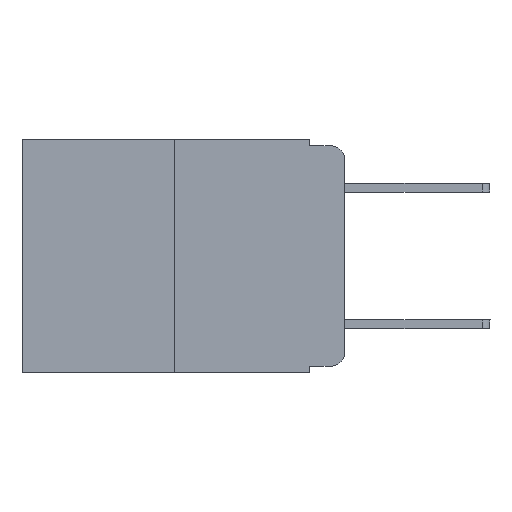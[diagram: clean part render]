
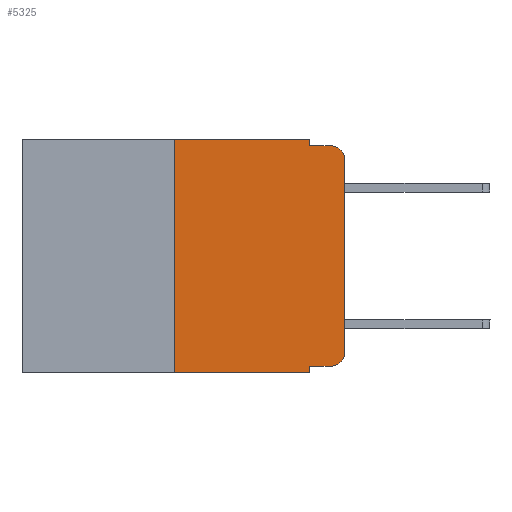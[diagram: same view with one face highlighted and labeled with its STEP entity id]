
A CAD part, left-side view. The second image highlights one B-rep face of the part: STEP entity #5325.
In plain terms, the highlighted planar face has unit normal (-1, 0, 0).
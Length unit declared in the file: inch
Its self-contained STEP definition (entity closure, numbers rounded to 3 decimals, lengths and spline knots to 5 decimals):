
#109 = DIRECTION ( 'NONE',  ( 0., 0., -1. ) ) ;
#669 = DIRECTION ( 'NONE',  ( 1., 0., 0. ) ) ;
#818 = DIRECTION ( 'NONE',  ( -1., 0., 0. ) ) ;
#1307 = AXIS2_PLACEMENT_3D ( 'NONE', #4629, #669, #14465 ) ;
#1633 = DIRECTION ( 'NONE',  ( 0., 0., 1. ) ) ;
#1715 = CARTESIAN_POINT ( 'NONE',  ( 0., 0.25, 0. ) ) ;
#1912 = EDGE_CURVE ( 'NONE', #17493, #9407, #16410, .T. ) ;
#2151 = AXIS2_PLACEMENT_3D ( 'NONE', #16665, #11224, #109 ) ;
#2293 = EDGE_CURVE ( 'NONE', #14883, #9252, #6086, .T. ) ;
#2622 = ORIENTED_EDGE ( 'NONE', *, *, #1912, .T. ) ;
#2721 = VERTEX_POINT ( 'NONE', #11916 ) ;
#2787 = DIRECTION ( 'NONE',  ( 0., -1., 0. ) ) ;
#2846 = VECTOR ( 'NONE', #4198, 39.37008 ) ;
#2857 = ORIENTED_EDGE ( 'NONE', *, *, #6611, .F. ) ;
#3054 = CARTESIAN_POINT ( 'NONE',  ( 0., 0.051, -0.343 ) ) ;
#3123 = LINE ( 'NONE', #12348, #15602 ) ;
#3141 = EDGE_CURVE ( 'NONE', #12394, #9407, #14872, .T. ) ;
#3648 = DIRECTION ( 'NONE',  ( 0., -1., 0. ) ) ;
#3745 = CARTESIAN_POINT ( 'NONE',  ( 0., 0.02, -0.333 ) ) ;
#3758 = VERTEX_POINT ( 'NONE', #16646 ) ;
#3773 = CARTESIAN_POINT ( 'NONE',  ( 0., 0.051, -0.333 ) ) ;
#4007 = DIRECTION ( 'NONE',  ( 0., -1., 0. ) ) ;
#4198 = DIRECTION ( 'NONE',  ( 0., 0., 1. ) ) ;
#4251 = CARTESIAN_POINT ( 'NONE',  ( 0., 0.051, -0.01 ) ) ;
#4394 = LINE ( 'NONE', #17704, #8910 ) ;
#4629 = CARTESIAN_POINT ( 'NONE',  ( 0., 0.473, 0. ) ) ;
#4828 = VECTOR ( 'NONE', #2787, 39.37008 ) ;
#4903 = DIRECTION ( 'NONE',  ( 0., 0., -1. ) ) ;
#4929 = CARTESIAN_POINT ( 'NONE',  ( 0., 0.02, -0.03 ) ) ;
#5201 = VERTEX_POINT ( 'NONE', #3054 ) ;
#5233 = CARTESIAN_POINT ( 'NONE',  ( 0., 0., -0.313 ) ) ;
#5248 = DIRECTION ( 'NONE',  ( 0., 0., -1. ) ) ;
#5325 = ADVANCED_FACE ( 'NONE', ( #15027 ), #16827, .F. ) ;
#6073 = VECTOR ( 'NONE', #4903, 39.37008 ) ;
#6086 = CIRCLE ( 'NONE', #2151, 0.02 ) ;
#6223 = EDGE_CURVE ( 'NONE', #9252, #17493, #13620, .T. ) ;
#6611 = EDGE_CURVE ( 'NONE', #11410, #5201, #9726, .T. ) ;
#6849 = CARTESIAN_POINT ( 'NONE',  ( 0., 0.02, -0.01 ) ) ;
#7162 = ORIENTED_EDGE ( 'NONE', *, *, #2293, .T. ) ;
#7163 = EDGE_LOOP ( 'NONE', ( #17812, #2622, #7362, #13199, #15242, #15354, #7691, #2857, #11344, #7162 ) ) ;
#7344 = CARTESIAN_POINT ( 'NONE',  ( 0., 0., -0.03 ) ) ;
#7362 = ORIENTED_EDGE ( 'NONE', *, *, #3141, .F. ) ;
#7691 = ORIENTED_EDGE ( 'NONE', *, *, #17057, .T. ) ;
#7762 = VECTOR ( 'NONE', #3648, 39.37008 ) ;
#7918 = CARTESIAN_POINT ( 'NONE',  ( 0., 0.051, 0. ) ) ;
#8222 = CARTESIAN_POINT ( 'NONE',  ( 0., 0., 0. ) ) ;
#8263 = LINE ( 'NONE', #9940, #10872 ) ;
#8910 = VECTOR ( 'NONE', #4007, 39.37008 ) ;
#9252 = VERTEX_POINT ( 'NONE', #5233 ) ;
#9407 = VERTEX_POINT ( 'NONE', #6849 ) ;
#9524 = VERTEX_POINT ( 'NONE', #1715 ) ;
#9726 = LINE ( 'NONE', #7918, #6073 ) ;
#9807 = CARTESIAN_POINT ( 'NONE',  ( 0., 0.051, -0.333 ) ) ;
#9940 = CARTESIAN_POINT ( 'NONE',  ( 0., 0.25, 0. ) ) ;
#10465 = DIRECTION ( 'NONE',  ( 0., 0., -1. ) ) ;
#10505 = CARTESIAN_POINT ( 'NONE',  ( 0., 0.051, -0.01 ) ) ;
#10703 = EDGE_CURVE ( 'NONE', #9524, #2721, #3123, .T. ) ;
#10872 = VECTOR ( 'NONE', #1633, 39.37008 ) ;
#10989 = LINE ( 'NONE', #12167, #15920 ) ;
#11224 = DIRECTION ( 'NONE',  ( -1., 0., 0. ) ) ;
#11344 = ORIENTED_EDGE ( 'NONE', *, *, #17165, .T. ) ;
#11410 = VERTEX_POINT ( 'NONE', #9807 ) ;
#11916 = CARTESIAN_POINT ( 'NONE',  ( 0., 0.051, 0. ) ) ;
#12167 = CARTESIAN_POINT ( 'NONE',  ( 0., 0.051, 0. ) ) ;
#12348 = CARTESIAN_POINT ( 'NONE',  ( 0., 0.473, 0. ) ) ;
#12394 = VERTEX_POINT ( 'NONE', #4251 ) ;
#12459 = EDGE_CURVE ( 'NONE', #3758, #9524, #8263, .T. ) ;
#13199 = ORIENTED_EDGE ( 'NONE', *, *, #13992, .F. ) ;
#13620 = LINE ( 'NONE', #8222, #2846 ) ;
#13992 = EDGE_CURVE ( 'NONE', #2721, #12394, #10989, .T. ) ;
#14465 = DIRECTION ( 'NONE',  ( 0., 0., -1. ) ) ;
#14735 = AXIS2_PLACEMENT_3D ( 'NONE', #4929, #818, #10465 ) ;
#14872 = LINE ( 'NONE', #10505, #7762 ) ;
#14883 = VERTEX_POINT ( 'NONE', #3745 ) ;
#15027 = FACE_OUTER_BOUND ( 'NONE', #7163, .T. ) ;
#15242 = ORIENTED_EDGE ( 'NONE', *, *, #10703, .F. ) ;
#15354 = ORIENTED_EDGE ( 'NONE', *, *, #12459, .F. ) ;
#15602 = VECTOR ( 'NONE', #17638, 39.37008 ) ;
#15920 = VECTOR ( 'NONE', #5248, 39.37008 ) ;
#16410 = CIRCLE ( 'NONE', #14735, 0.02 ) ;
#16646 = CARTESIAN_POINT ( 'NONE',  ( 0., 0.25, -0.343 ) ) ;
#16665 = CARTESIAN_POINT ( 'NONE',  ( 0., 0.02, -0.313 ) ) ;
#16827 = PLANE ( 'NONE',  #1307 ) ;
#17057 = EDGE_CURVE ( 'NONE', #3758, #5201, #4394, .T. ) ;
#17077 = LINE ( 'NONE', #3773, #4828 ) ;
#17165 = EDGE_CURVE ( 'NONE', #11410, #14883, #17077, .T. ) ;
#17493 = VERTEX_POINT ( 'NONE', #7344 ) ;
#17638 = DIRECTION ( 'NONE',  ( 0., -1., 0. ) ) ;
#17704 = CARTESIAN_POINT ( 'NONE',  ( 0., 0.473, -0.343 ) ) ;
#17812 = ORIENTED_EDGE ( 'NONE', *, *, #6223, .T. ) ;
